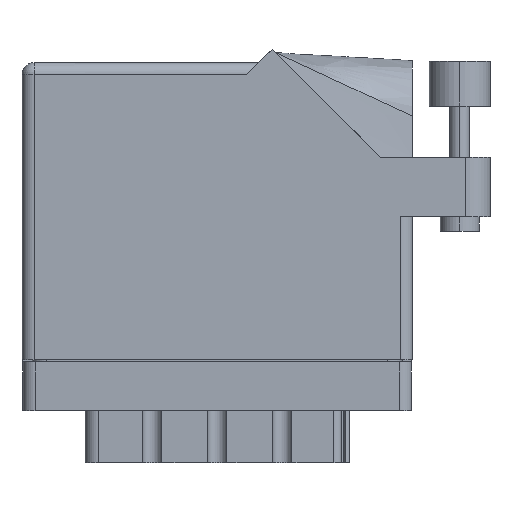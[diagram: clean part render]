
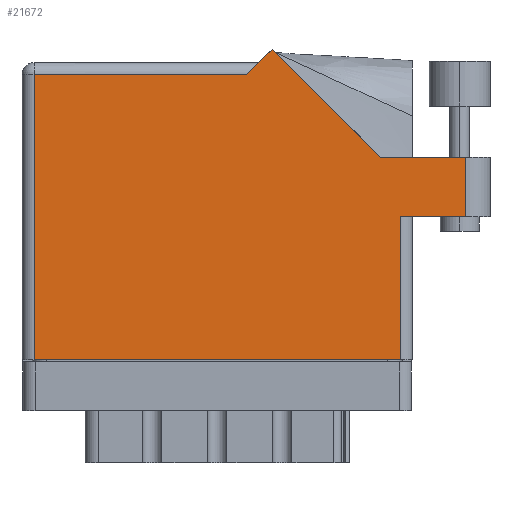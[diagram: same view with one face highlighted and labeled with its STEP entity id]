
A CAD part, front view. The second image highlights one B-rep face of the part: STEP entity #21672.
In plain terms, the highlighted face is planar.
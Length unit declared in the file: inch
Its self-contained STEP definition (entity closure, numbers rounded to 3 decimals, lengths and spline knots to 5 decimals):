
#526 = EDGE_CURVE ( 'NONE', #1829, #13812, #9112, .T. ) ;
#768 = CARTESIAN_POINT ( 'NONE',  ( 0.062, 0., 0. ) ) ;
#799 = ORIENTED_EDGE ( 'NONE', *, *, #14247, .T. ) ;
#1169 = CARTESIAN_POINT ( 'NONE',  ( 2.285, 0.737, 0. ) ) ;
#1829 = VERTEX_POINT ( 'NONE', #7052 ) ;
#1989 = LINE ( 'NONE', #768, #14538 ) ;
#2433 = LINE ( 'NONE', #25975, #25254 ) ;
#2761 = CARTESIAN_POINT ( 'NONE',  ( 0.062, 0., 0. ) ) ;
#3031 = FACE_OUTER_BOUND ( 'NONE', #5134, .T. ) ;
#3424 = VERTEX_POINT ( 'NONE', #1169 ) ;
#3508 = CARTESIAN_POINT ( 'NONE',  ( 0., 1.53, 0. ) ) ;
#4147 = CARTESIAN_POINT ( 'NONE',  ( 2.285, 1.044, 0. ) ) ;
#4884 = VERTEX_POINT ( 'NONE', #4147 ) ;
#5134 = EDGE_LOOP ( 'NONE', ( #799, #11203, #35821, #30576, #29415, #20130, #13774, #13180, #33515 ) ) ;
#5991 = DIRECTION ( 'NONE',  ( 0., 1., 0. ) ) ;
#6129 = DIRECTION ( 'NONE',  ( 1., 0., 0. ) ) ;
#6576 = DIRECTION ( 'NONE',  ( 0., -1., 0. ) ) ;
#7052 = CARTESIAN_POINT ( 'NONE',  ( 1.155, 1.468, 0. ) ) ;
#7698 = CARTESIAN_POINT ( 'NONE',  ( 1.84442, 1.044, 0. ) ) ;
#9112 = LINE ( 'NONE', #14651, #24803 ) ;
#9227 = LINE ( 'NONE', #27971, #23539 ) ;
#10427 = CARTESIAN_POINT ( 'NONE',  ( 2.41, 1.044, 0. ) ) ;
#11203 = ORIENTED_EDGE ( 'NONE', *, *, #33871, .T. ) ;
#11255 = LINE ( 'NONE', #10427, #33248 ) ;
#11591 = VERTEX_POINT ( 'NONE', #36340 ) ;
#11861 = CARTESIAN_POINT ( 'NONE',  ( 2.285, 1.044, 0. ) ) ;
#13180 = ORIENTED_EDGE ( 'NONE', *, *, #29102, .T. ) ;
#13774 = ORIENTED_EDGE ( 'NONE', *, *, #24505, .T. ) ;
#13812 = VERTEX_POINT ( 'NONE', #19048 ) ;
#13898 = VERTEX_POINT ( 'NONE', #2761 ) ;
#14247 = EDGE_CURVE ( 'NONE', #11591, #3424, #15466, .T. ) ;
#14538 = VECTOR ( 'NONE', #6576, 39.37008 ) ;
#14651 = CARTESIAN_POINT ( 'NONE',  ( 0., 1.468, 0. ) ) ;
#14750 = DIRECTION ( 'NONE',  ( 0., 1., 0. ) ) ;
#15466 = LINE ( 'NONE', #34360, #32088 ) ;
#17174 = DIRECTION ( 'NONE',  ( 1., 0., 0. ) ) ;
#17791 = CARTESIAN_POINT ( 'NONE',  ( 1.217, 1.53, 0. ) ) ;
#18270 = VERTEX_POINT ( 'NONE', #21354 ) ;
#18835 = LINE ( 'NONE', #26122, #34541 ) ;
#19048 = CARTESIAN_POINT ( 'NONE',  ( 0.062, 1.468, 0. ) ) ;
#20130 = ORIENTED_EDGE ( 'NONE', *, *, #526, .T. ) ;
#20936 = CARTESIAN_POINT ( 'NONE',  ( 1.948, 0., 0. ) ) ;
#21354 = CARTESIAN_POINT ( 'NONE',  ( 1.28771, 1.60071, 0. ) ) ;
#21672 = ADVANCED_FACE ( 'NONE', ( #3031 ), #29282, .F. ) ;
#21940 = DIRECTION ( 'NONE',  ( -1., 0., 0. ) ) ;
#23011 = EDGE_CURVE ( 'NONE', #18270, #1829, #31257, .T. ) ;
#23392 = DIRECTION ( 'NONE',  ( 0., 0., -1. ) ) ;
#23539 = VECTOR ( 'NONE', #25459, 39.37008 ) ;
#24505 = EDGE_CURVE ( 'NONE', #13812, #13898, #1989, .T. ) ;
#24803 = VECTOR ( 'NONE', #34594, 39.37008 ) ;
#25254 = VECTOR ( 'NONE', #5991, 39.37008 ) ;
#25459 = DIRECTION ( 'NONE',  ( -0.707, 0.707, 0. ) ) ;
#25975 = CARTESIAN_POINT ( 'NONE',  ( 1.948, 0.737, 0. ) ) ;
#26122 = CARTESIAN_POINT ( 'NONE',  ( 0., 0., 0. ) ) ;
#26298 = DIRECTION ( 'NONE',  ( -0.707, -0.707, 0. ) ) ;
#26403 = VERTEX_POINT ( 'NONE', #7698 ) ;
#26467 = EDGE_CURVE ( 'NONE', #4884, #26403, #11255, .T. ) ;
#26768 = AXIS2_PLACEMENT_3D ( 'NONE', #3508, #23392, #31824 ) ;
#27971 = CARTESIAN_POINT ( 'NONE',  ( 1.84442, 1.044, 0. ) ) ;
#28806 = VECTOR ( 'NONE', #14750, 39.37008 ) ;
#29102 = EDGE_CURVE ( 'NONE', #13898, #33416, #18835, .T. ) ;
#29282 = PLANE ( 'NONE',  #26768 ) ;
#29415 = ORIENTED_EDGE ( 'NONE', *, *, #23011, .T. ) ;
#29900 = VECTOR ( 'NONE', #26298, 39.37008 ) ;
#30576 = ORIENTED_EDGE ( 'NONE', *, *, #32616, .T. ) ;
#31257 = LINE ( 'NONE', #17791, #29900 ) ;
#31824 = DIRECTION ( 'NONE',  ( -1., 0., 0. ) ) ;
#32088 = VECTOR ( 'NONE', #17174, 39.37008 ) ;
#32616 = EDGE_CURVE ( 'NONE', #26403, #18270, #9227, .T. ) ;
#33248 = VECTOR ( 'NONE', #21940, 39.37008 ) ;
#33361 = LINE ( 'NONE', #11861, #28806 ) ;
#33416 = VERTEX_POINT ( 'NONE', #20936 ) ;
#33515 = ORIENTED_EDGE ( 'NONE', *, *, #36284, .T. ) ;
#33871 = EDGE_CURVE ( 'NONE', #3424, #4884, #33361, .T. ) ;
#34360 = CARTESIAN_POINT ( 'NONE',  ( 2.01, 0.737, 0. ) ) ;
#34541 = VECTOR ( 'NONE', #6129, 39.37008 ) ;
#34594 = DIRECTION ( 'NONE',  ( -1., 0., 0. ) ) ;
#35821 = ORIENTED_EDGE ( 'NONE', *, *, #26467, .T. ) ;
#36284 = EDGE_CURVE ( 'NONE', #33416, #11591, #2433, .T. ) ;
#36340 = CARTESIAN_POINT ( 'NONE',  ( 1.948, 0.737, 0. ) ) ;
